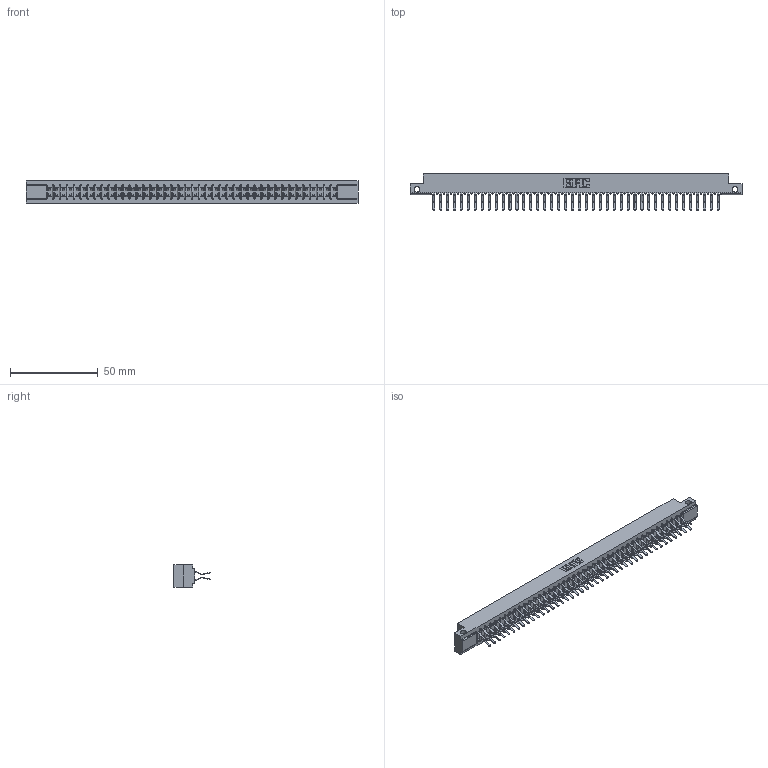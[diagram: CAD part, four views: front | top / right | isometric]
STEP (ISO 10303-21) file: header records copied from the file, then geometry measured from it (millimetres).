
FILE_DESCRIPTION (( 'STEP AP203' ), '1' );
FILE_NAME ('307-084-460-212.STEP', '2020-10-01T13:21:15', ( '' ), ( '' ), 'SwSTEP 2.0', 'SolidWorks 2020', '' );
FILE_SCHEMA (( 'CONFIG_CONTROL_DESIGN' ));
Length unit declared in the file: inch
Products named in the file (3): 307-084-460-212; 307-290-001_560; 307 Part_.128 Dia Side Mounting Holes
Assembly tree (85 placements, depth 2):
  307-084-460-212
    307 Part_.128 Dia Side Mounting Holes
    307-290-001_560  x84
Bounding box: 189.43 x 20.73 x 12.7 mm (x, y, z)
Volume: 20106.6 mm3; surface area: 25150.7 mm2
Topology: 85 solids, 85 shells, 4361 faces, 12251 edges, 7938 vertices
Faces by surface type: plane 2842, cylinder 1433, sphere 86
Entity records: 37456 total; most frequent: CARTESIAN_POINT 6126, ORIENTED_EDGE 6070, DIRECTION 6001, EDGE_CURVE 3035, VECTOR 2327, LINE 2327, VERTEX_POINT 1962, AXIS2_PLACEMENT_3D 1837
